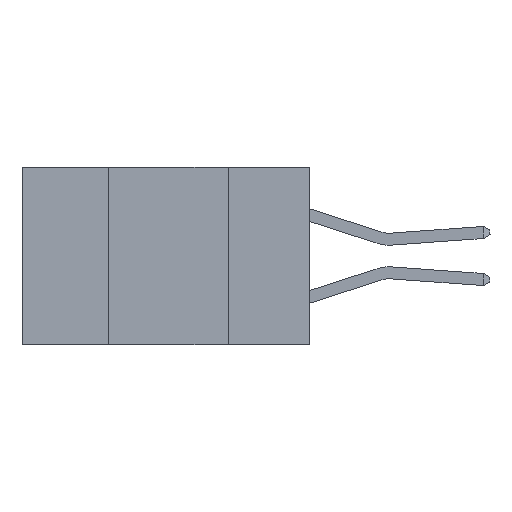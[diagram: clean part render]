
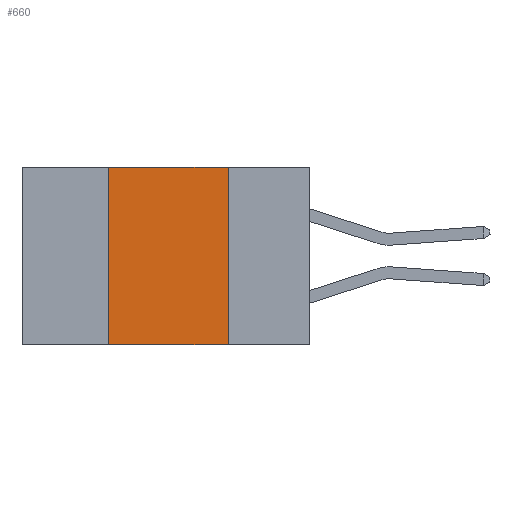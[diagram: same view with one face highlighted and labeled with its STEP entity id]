
A CAD part, left-side view. The second image highlights one B-rep face of the part: STEP entity #660.
In plain terms, the highlighted planar face has unit normal (-1, 0, 0).
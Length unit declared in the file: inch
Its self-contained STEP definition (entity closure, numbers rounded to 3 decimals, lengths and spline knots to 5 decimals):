
#380 = CARTESIAN_POINT ( 'NONE',  ( 0., 0.42, 0. ) ) ;
#412 = CARTESIAN_POINT ( 'NONE',  ( 0., 0.6, 0. ) ) ;
#660 = ADVANCED_FACE ( 'NONE', ( #1125 ), #11214, .F. ) ;
#944 = EDGE_CURVE ( 'NONE', #11520, #11775, #10105, .T. ) ;
#1125 = FACE_OUTER_BOUND ( 'NONE', #2532, .T. ) ;
#2140 = ORIENTED_EDGE ( 'NONE', *, *, #7822, .F. ) ;
#2532 = EDGE_LOOP ( 'NONE', ( #9316, #2140, #11574, #4086 ) ) ;
#2579 = LINE ( 'NONE', #5844, #11533 ) ;
#3421 = VERTEX_POINT ( 'NONE', #380 ) ;
#3812 = VERTEX_POINT ( 'NONE', #10096 ) ;
#3976 = VECTOR ( 'NONE', #10539, 39.37008 ) ;
#4086 = ORIENTED_EDGE ( 'NONE', *, *, #944, .T. ) ;
#5206 = DIRECTION ( 'NONE',  ( 0., -1., 0. ) ) ;
#5408 = VECTOR ( 'NONE', #5206, 39.37008 ) ;
#5608 = DIRECTION ( 'NONE',  ( 0., -1., 0. ) ) ;
#5844 = CARTESIAN_POINT ( 'NONE',  ( 0., 0.6, 0. ) ) ;
#5923 = CARTESIAN_POINT ( 'NONE',  ( 0., 0.17, -0.37 ) ) ;
#6096 = DIRECTION ( 'NONE',  ( 0., 0., -1. ) ) ;
#6113 = DIRECTION ( 'NONE',  ( 1., 0., 0. ) ) ;
#6517 = LINE ( 'NONE', #10552, #3976 ) ;
#7295 = VECTOR ( 'NONE', #9824, 39.37008 ) ;
#7644 = CARTESIAN_POINT ( 'NONE',  ( 0., 0.42, -0.37 ) ) ;
#7822 = EDGE_CURVE ( 'NONE', #3421, #3812, #2579, .T. ) ;
#8277 = EDGE_CURVE ( 'NONE', #3812, #11775, #9411, .T. ) ;
#9316 = ORIENTED_EDGE ( 'NONE', *, *, #8277, .F. ) ;
#9411 = LINE ( 'NONE', #9781, #7295 ) ;
#9417 = AXIS2_PLACEMENT_3D ( 'NONE', #412, #6113, #6096 ) ;
#9781 = CARTESIAN_POINT ( 'NONE',  ( 0., 0.17, -0.37 ) ) ;
#9824 = DIRECTION ( 'NONE',  ( 0., 0., -1. ) ) ;
#10096 = CARTESIAN_POINT ( 'NONE',  ( 0., 0.17, 0. ) ) ;
#10105 = LINE ( 'NONE', #10222, #5408 ) ;
#10222 = CARTESIAN_POINT ( 'NONE',  ( 0., 0.6, -0.37 ) ) ;
#10539 = DIRECTION ( 'NONE',  ( 0., 0., 1. ) ) ;
#10552 = CARTESIAN_POINT ( 'NONE',  ( 0., 0.42, -0.37 ) ) ;
#11112 = EDGE_CURVE ( 'NONE', #11520, #3421, #6517, .T. ) ;
#11214 = PLANE ( 'NONE',  #9417 ) ;
#11520 = VERTEX_POINT ( 'NONE', #7644 ) ;
#11533 = VECTOR ( 'NONE', #5608, 39.37008 ) ;
#11574 = ORIENTED_EDGE ( 'NONE', *, *, #11112, .F. ) ;
#11775 = VERTEX_POINT ( 'NONE', #5923 ) ;
